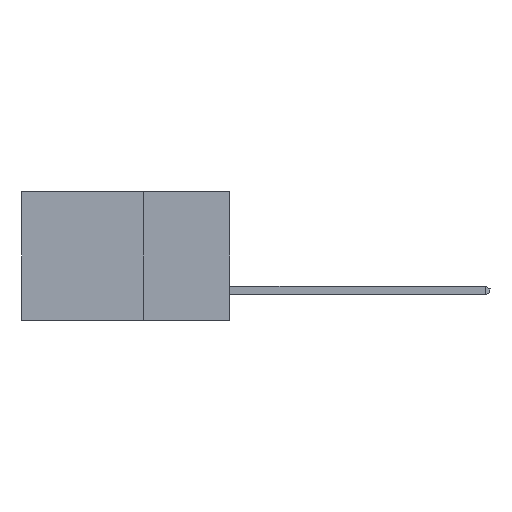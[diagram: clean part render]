
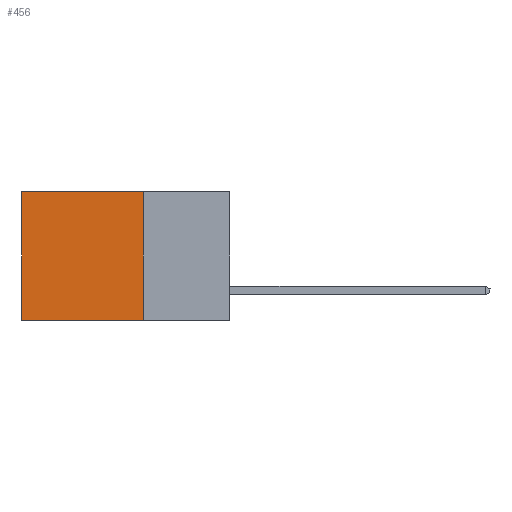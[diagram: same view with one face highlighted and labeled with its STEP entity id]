
A CAD part, left-side view. The second image highlights one B-rep face of the part: STEP entity #456.
In plain terms, the highlighted planar face has unit normal (-1, 0, 0).
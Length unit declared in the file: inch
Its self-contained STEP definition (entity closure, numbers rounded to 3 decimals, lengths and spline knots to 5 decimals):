
#456 = ADVANCED_FACE ( 'NONE', ( #15967 ), #12010, .F. ) ;
#660 = ORIENTED_EDGE ( 'NONE', *, *, #14809, .T. ) ;
#940 = DIRECTION ( 'NONE',  ( 0., 0., -1. ) ) ;
#987 = AXIS2_PLACEMENT_3D ( 'NONE', #7935, #17214, #7994 ) ;
#1190 = DIRECTION ( 'NONE',  ( 0., 0., -1. ) ) ;
#1709 = EDGE_CURVE ( 'NONE', #13273, #8450, #2633, .T. ) ;
#2222 = DIRECTION ( 'NONE',  ( 0., 1., 0. ) ) ;
#2477 = VERTEX_POINT ( 'NONE', #15261 ) ;
#2633 = LINE ( 'NONE', #2751, #8738 ) ;
#2751 = CARTESIAN_POINT ( 'NONE',  ( 0.298, 0.6, 0. ) ) ;
#3710 = CARTESIAN_POINT ( 'NONE',  ( 0.298, 0.6, -0.37 ) ) ;
#3716 = EDGE_LOOP ( 'NONE', ( #7144, #10634, #10698, #660 ) ) ;
#3888 = EDGE_CURVE ( 'NONE', #16405, #8450, #7707, .T. ) ;
#3983 = CARTESIAN_POINT ( 'NONE',  ( 0.298, 0.25, 0. ) ) ;
#4151 = VECTOR ( 'NONE', #9631, 39.37008 ) ;
#6774 = VECTOR ( 'NONE', #1190, 39.37008 ) ;
#6885 = CARTESIAN_POINT ( 'NONE',  ( 0.298, 0.25, -0.37 ) ) ;
#7144 = ORIENTED_EDGE ( 'NONE', *, *, #1709, .T. ) ;
#7580 = CARTESIAN_POINT ( 'NONE',  ( 0.298, 0.25, 0. ) ) ;
#7707 = LINE ( 'NONE', #6885, #4151 ) ;
#7935 = CARTESIAN_POINT ( 'NONE',  ( 0.298, 0.25, 0. ) ) ;
#7994 = DIRECTION ( 'NONE',  ( 0., 0., -1. ) ) ;
#8450 = VERTEX_POINT ( 'NONE', #3710 ) ;
#8726 = CARTESIAN_POINT ( 'NONE',  ( 0.298, 0.6, 0. ) ) ;
#8738 = VECTOR ( 'NONE', #940, 39.37008 ) ;
#9631 = DIRECTION ( 'NONE',  ( 0., 1., 0. ) ) ;
#10634 = ORIENTED_EDGE ( 'NONE', *, *, #3888, .F. ) ;
#10698 = ORIENTED_EDGE ( 'NONE', *, *, #10939, .F. ) ;
#10939 = EDGE_CURVE ( 'NONE', #2477, #16405, #13733, .T. ) ;
#12010 = PLANE ( 'NONE',  #987 ) ;
#12291 = CARTESIAN_POINT ( 'NONE',  ( 0.298, 0.25, -0.37 ) ) ;
#13273 = VERTEX_POINT ( 'NONE', #8726 ) ;
#13733 = LINE ( 'NONE', #3983, #6774 ) ;
#14809 = EDGE_CURVE ( 'NONE', #2477, #13273, #15927, .T. ) ;
#15261 = CARTESIAN_POINT ( 'NONE',  ( 0.298, 0.25, 0. ) ) ;
#15507 = VECTOR ( 'NONE', #2222, 39.37008 ) ;
#15927 = LINE ( 'NONE', #7580, #15507 ) ;
#15967 = FACE_OUTER_BOUND ( 'NONE', #3716, .T. ) ;
#16405 = VERTEX_POINT ( 'NONE', #12291 ) ;
#17214 = DIRECTION ( 'NONE',  ( 1., 0., 0. ) ) ;
